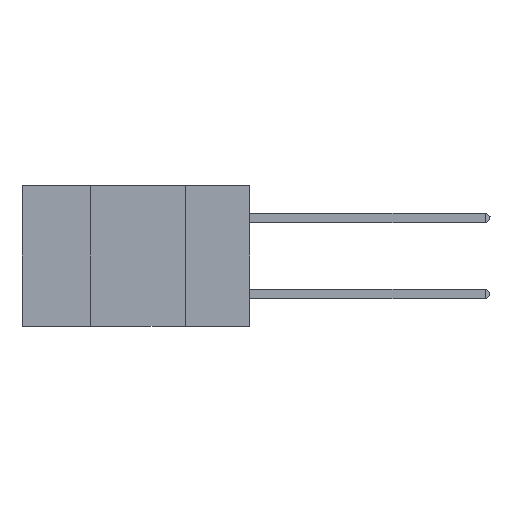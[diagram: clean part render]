
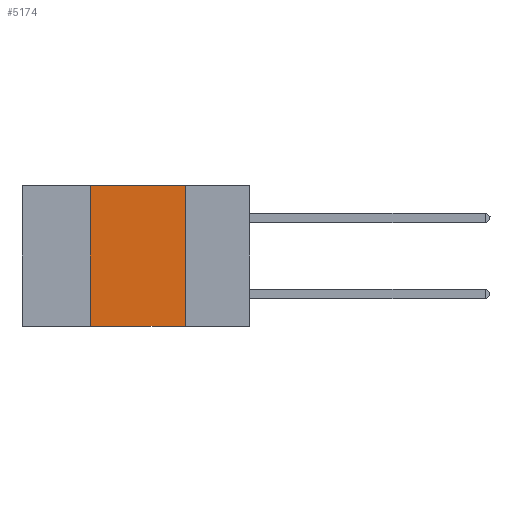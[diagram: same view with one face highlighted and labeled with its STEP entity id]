
A CAD part, left-side view. The second image highlights one B-rep face of the part: STEP entity #5174.
In plain terms, the highlighted planar face has unit normal (-1, 0, 0).
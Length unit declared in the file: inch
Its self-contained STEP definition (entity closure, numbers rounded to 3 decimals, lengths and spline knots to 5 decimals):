
#153 = CARTESIAN_POINT ( 'NONE',  ( 0., 0.42, 0. ) ) ;
#291 = ORIENTED_EDGE ( 'NONE', *, *, #10114, .T. ) ;
#537 = AXIS2_PLACEMENT_3D ( 'NONE', #11385, #749, #9135 ) ;
#749 = DIRECTION ( 'NONE',  ( 1., 0., 0. ) ) ;
#1489 = VECTOR ( 'NONE', #12420, 39.37008 ) ;
#1498 = VECTOR ( 'NONE', #8976, 39.37008 ) ;
#1897 = CARTESIAN_POINT ( 'NONE',  ( 0., 0.6, -0.37 ) ) ;
#1907 = PLANE ( 'NONE',  #537 ) ;
#2327 = CARTESIAN_POINT ( 'NONE',  ( 0., 0.17, -0.37 ) ) ;
#2677 = ORIENTED_EDGE ( 'NONE', *, *, #3352, .F. ) ;
#3141 = DIRECTION ( 'NONE',  ( 0., -1., 0. ) ) ;
#3352 = EDGE_CURVE ( 'NONE', #7348, #15329, #12107, .T. ) ;
#3615 = CARTESIAN_POINT ( 'NONE',  ( 0., 0.42, -0.37 ) ) ;
#4107 = CARTESIAN_POINT ( 'NONE',  ( 0., 0.42, 0. ) ) ;
#4563 = LINE ( 'NONE', #4797, #5755 ) ;
#4797 = CARTESIAN_POINT ( 'NONE',  ( 0., 0.17, 0. ) ) ;
#4850 = VERTEX_POINT ( 'NONE', #11960 ) ;
#4874 = ORIENTED_EDGE ( 'NONE', *, *, #5256, .F. ) ;
#5159 = EDGE_CURVE ( 'NONE', #15329, #4850, #6896, .T. ) ;
#5174 = ADVANCED_FACE ( 'NONE', ( #7828 ), #1907, .F. ) ;
#5256 = EDGE_CURVE ( 'NONE', #4850, #6136, #4563, .T. ) ;
#5755 = VECTOR ( 'NONE', #9814, 39.37008 ) ;
#6136 = VERTEX_POINT ( 'NONE', #2327 ) ;
#6896 = LINE ( 'NONE', #9065, #10209 ) ;
#7348 = VERTEX_POINT ( 'NONE', #3615 ) ;
#7828 = FACE_OUTER_BOUND ( 'NONE', #9145, .T. ) ;
#8976 = DIRECTION ( 'NONE',  ( 0., -1., 0. ) ) ;
#9065 = CARTESIAN_POINT ( 'NONE',  ( 0., 0.6, 0. ) ) ;
#9135 = DIRECTION ( 'NONE',  ( 0., 0., -1. ) ) ;
#9145 = EDGE_LOOP ( 'NONE', ( #4874, #13893, #2677, #291 ) ) ;
#9814 = DIRECTION ( 'NONE',  ( 0., 0., -1. ) ) ;
#10114 = EDGE_CURVE ( 'NONE', #7348, #6136, #13793, .T. ) ;
#10209 = VECTOR ( 'NONE', #3141, 39.37008 ) ;
#11385 = CARTESIAN_POINT ( 'NONE',  ( 0., 0.6, 0. ) ) ;
#11960 = CARTESIAN_POINT ( 'NONE',  ( 0., 0.17, 0. ) ) ;
#12107 = LINE ( 'NONE', #4107, #1489 ) ;
#12420 = DIRECTION ( 'NONE',  ( 0., 0., 1. ) ) ;
#13793 = LINE ( 'NONE', #1897, #1498 ) ;
#13893 = ORIENTED_EDGE ( 'NONE', *, *, #5159, .F. ) ;
#15329 = VERTEX_POINT ( 'NONE', #153 ) ;
